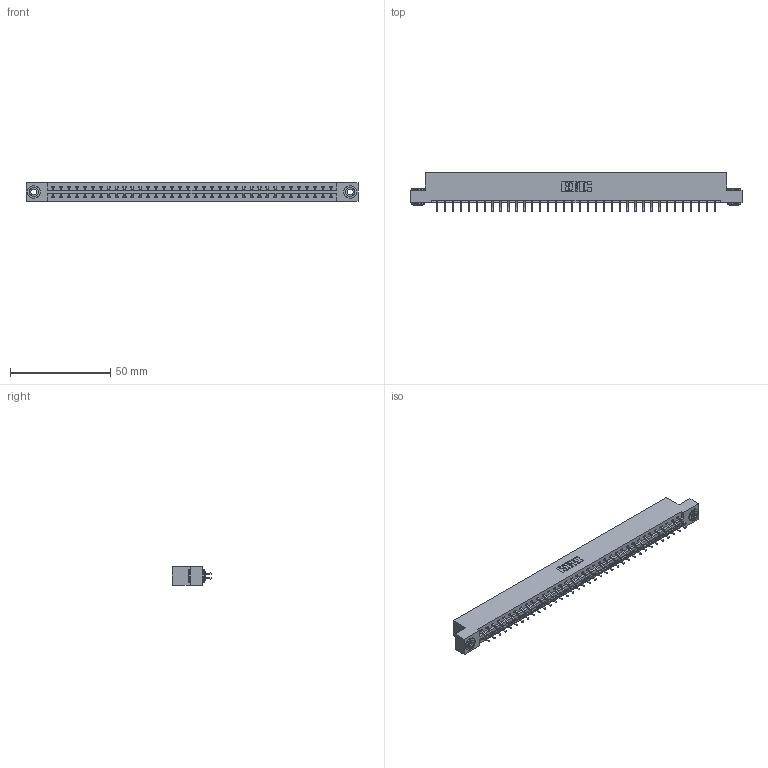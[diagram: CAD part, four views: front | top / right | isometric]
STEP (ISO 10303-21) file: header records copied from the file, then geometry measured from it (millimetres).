
FILE_DESCRIPTION (( 'STEP AP203' ), '1' );
FILE_NAME ('387-072-556-203.STEP', '2018-09-22T18:44:11', ( '' ), ( '' ), 'SwSTEP 2.0', 'SolidWorks 2016', '' );
FILE_SCHEMA (( 'CONFIG_CONTROL_DESIGN' ));
Length unit declared in the file: inch
Products named in the file (4): 345-292-001_556 Tail; 345-250-002_345-250-002-102; 387-072-556-203; 337 Part_Flush Mounting Lugs - 0.156 Dia-TH
Assembly tree (75 placements, depth 2):
  387-072-556-203
    337 Part_Flush Mounting Lugs - 0.156 Dia-TH
    345-292-001_556 Tail  x72
    345-250-002_345-250-002-102  x2
Bounding box: 165.66 x 19.57 x 9.4 mm (x, y, z)
Volume: 17395.1 mm3; surface area: 19755.4 mm2
Topology: 75 solids, 75 shells, 4472 faces, 13275 edges, 8750 vertices
Faces by surface type: plane 3104, cylinder 1360, cone 8
Entity records: 29558 total; most frequent: CARTESIAN_POINT 4973, ORIENTED_EDGE 4890, DIRECTION 4263, EDGE_CURVE 2445, VECTOR 2285, LINE 2285, VERTEX_POINT 1626, AXIS2_PLACEMENT_3D 989
